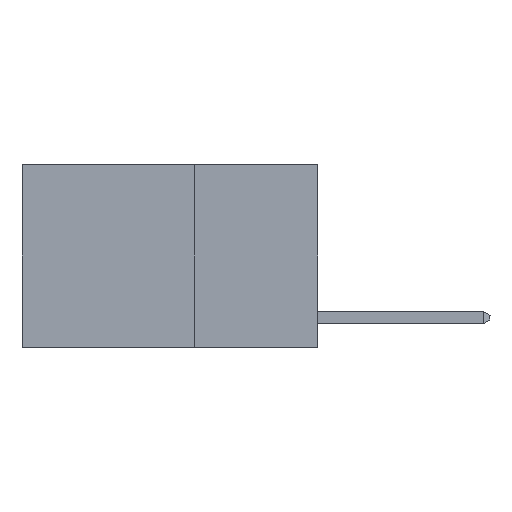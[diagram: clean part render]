
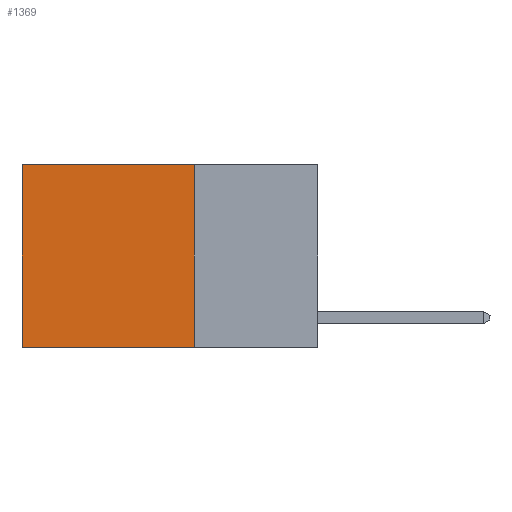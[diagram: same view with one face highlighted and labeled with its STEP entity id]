
A CAD part, left-side view. The second image highlights one B-rep face of the part: STEP entity #1369.
In plain terms, the highlighted planar face has unit normal (-1, 0, 0).
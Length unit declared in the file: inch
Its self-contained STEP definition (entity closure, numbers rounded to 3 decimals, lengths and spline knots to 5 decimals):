
#448 = EDGE_CURVE ( 'NONE', #6897, #4279, #6151, .T. ) ;
#1046 = LINE ( 'NONE', #4857, #7230 ) ;
#1168 = FACE_OUTER_BOUND ( 'NONE', #8017, .T. ) ;
#1369 = ADVANCED_FACE ( 'NONE', ( #1168 ), #15467, .F. ) ;
#1687 = VECTOR ( 'NONE', #9996, 39.37008 ) ;
#1932 = ORIENTED_EDGE ( 'NONE', *, *, #13872, .F. ) ;
#2243 = ORIENTED_EDGE ( 'NONE', *, *, #448, .T. ) ;
#2596 = ORIENTED_EDGE ( 'NONE', *, *, #2757, .T. ) ;
#2757 = EDGE_CURVE ( 'NONE', #12757, #6897, #1046, .T. ) ;
#3967 = CARTESIAN_POINT ( 'NONE',  ( 0.2625, 0.25, 0. ) ) ;
#4229 = EDGE_CURVE ( 'NONE', #12757, #12641, #11257, .T. ) ;
#4279 = VERTEX_POINT ( 'NONE', #6855 ) ;
#4644 = CARTESIAN_POINT ( 'NONE',  ( 0.2625, 0.6, 0. ) ) ;
#4795 = CARTESIAN_POINT ( 'NONE',  ( 0.2625, 0.25, 0. ) ) ;
#4857 = CARTESIAN_POINT ( 'NONE',  ( 0.2625, 0.25, 0. ) ) ;
#5360 = VECTOR ( 'NONE', #13871, 39.37008 ) ;
#5833 = CARTESIAN_POINT ( 'NONE',  ( 0.2625, 0.25, -0.37 ) ) ;
#6151 = LINE ( 'NONE', #11427, #5360 ) ;
#6198 = DIRECTION ( 'NONE',  ( 0., 1., 0. ) ) ;
#6855 = CARTESIAN_POINT ( 'NONE',  ( 0.2625, 0.6, -0.37 ) ) ;
#6897 = VERTEX_POINT ( 'NONE', #4644 ) ;
#6942 = ORIENTED_EDGE ( 'NONE', *, *, #4229, .F. ) ;
#7230 = VECTOR ( 'NONE', #6198, 39.37008 ) ;
#7309 = DIRECTION ( 'NONE',  ( 0., 1., 0. ) ) ;
#8017 = EDGE_LOOP ( 'NONE', ( #2243, #1932, #6942, #2596 ) ) ;
#8516 = AXIS2_PLACEMENT_3D ( 'NONE', #12556, #13818, #13509 ) ;
#9996 = DIRECTION ( 'NONE',  ( 0., 0., -1. ) ) ;
#11257 = LINE ( 'NONE', #4795, #1687 ) ;
#11427 = CARTESIAN_POINT ( 'NONE',  ( 0.2625, 0.6, 0. ) ) ;
#12488 = LINE ( 'NONE', #16259, #14866 ) ;
#12556 = CARTESIAN_POINT ( 'NONE',  ( 0.2625, 0.25, 0. ) ) ;
#12641 = VERTEX_POINT ( 'NONE', #5833 ) ;
#12757 = VERTEX_POINT ( 'NONE', #3967 ) ;
#13509 = DIRECTION ( 'NONE',  ( 0., 0., -1. ) ) ;
#13818 = DIRECTION ( 'NONE',  ( 1., 0., 0. ) ) ;
#13871 = DIRECTION ( 'NONE',  ( 0., 0., -1. ) ) ;
#13872 = EDGE_CURVE ( 'NONE', #12641, #4279, #12488, .T. ) ;
#14866 = VECTOR ( 'NONE', #7309, 39.37008 ) ;
#15467 = PLANE ( 'NONE',  #8516 ) ;
#16259 = CARTESIAN_POINT ( 'NONE',  ( 0.2625, 0.25, -0.37 ) ) ;
